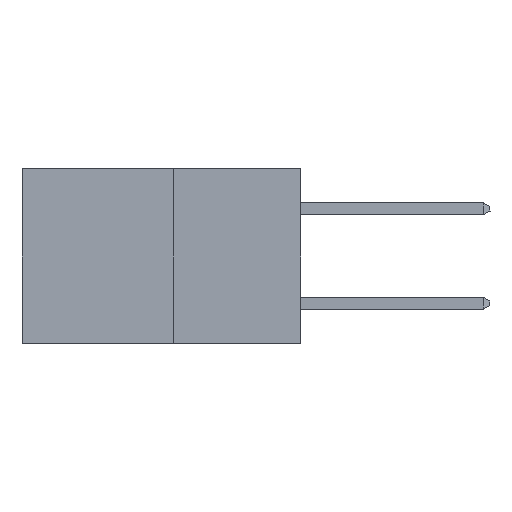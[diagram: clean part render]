
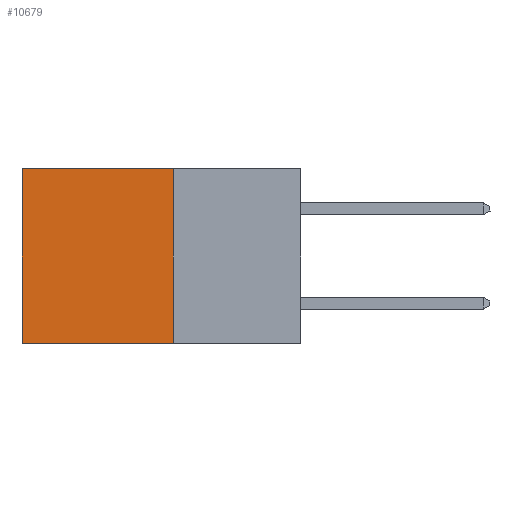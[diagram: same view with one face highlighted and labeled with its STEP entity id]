
A CAD part, left-side view. The second image highlights one B-rep face of the part: STEP entity #10679.
In plain terms, the highlighted planar face has unit normal (-1, 0, 0).
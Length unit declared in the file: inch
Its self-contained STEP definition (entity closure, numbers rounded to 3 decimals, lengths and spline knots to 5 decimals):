
#795 = DIRECTION ( 'NONE',  ( 0., 0., -1. ) ) ;
#1395 = LINE ( 'NONE', #13240, #25590 ) ;
#1588 = ORIENTED_EDGE ( 'NONE', *, *, #17756, .T. ) ;
#4269 = FACE_OUTER_BOUND ( 'NONE', #24309, .T. ) ;
#5501 = AXIS2_PLACEMENT_3D ( 'NONE', #5782, #15832, #795 ) ;
#5782 = CARTESIAN_POINT ( 'NONE',  ( 0.277, 0.27, -0.37 ) ) ;
#6312 = DIRECTION ( 'NONE',  ( 0., 0., -1. ) ) ;
#6482 = LINE ( 'NONE', #16261, #12352 ) ;
#6827 = EDGE_CURVE ( 'NONE', #15611, #18702, #25034, .T. ) ;
#7645 = DIRECTION ( 'NONE',  ( 0., 0., -1. ) ) ;
#8104 = CARTESIAN_POINT ( 'NONE',  ( 0.277, 0.27, -0.37 ) ) ;
#10357 = CARTESIAN_POINT ( 'NONE',  ( 0.277, 0.27, -0.37 ) ) ;
#10679 = ADVANCED_FACE ( 'NONE', ( #4269 ), #30623, .F. ) ;
#11931 = EDGE_CURVE ( 'NONE', #15611, #28631, #1395, .T. ) ;
#12152 = ORIENTED_EDGE ( 'NONE', *, *, #25305, .F. ) ;
#12352 = VECTOR ( 'NONE', #6312, 39.37008 ) ;
#13240 = CARTESIAN_POINT ( 'NONE',  ( 0.277, 0.27, 0. ) ) ;
#13281 = CARTESIAN_POINT ( 'NONE',  ( 0.277, 0.59, 0. ) ) ;
#15611 = VERTEX_POINT ( 'NONE', #28821 ) ;
#15832 = DIRECTION ( 'NONE',  ( 1., 0., 0. ) ) ;
#16261 = CARTESIAN_POINT ( 'NONE',  ( 0.277, 0.59, -0.37 ) ) ;
#17170 = VECTOR ( 'NONE', #20236, 39.37008 ) ;
#17756 = EDGE_CURVE ( 'NONE', #28631, #27104, #6482, .T. ) ;
#17958 = LINE ( 'NONE', #10357, #17170 ) ;
#18069 = ORIENTED_EDGE ( 'NONE', *, *, #11931, .T. ) ;
#18287 = DIRECTION ( 'NONE',  ( 0., 1., 0. ) ) ;
#18540 = ORIENTED_EDGE ( 'NONE', *, *, #6827, .F. ) ;
#18702 = VERTEX_POINT ( 'NONE', #24432 ) ;
#20011 = VECTOR ( 'NONE', #7645, 39.37008 ) ;
#20236 = DIRECTION ( 'NONE',  ( 0., 1., 0. ) ) ;
#24309 = EDGE_LOOP ( 'NONE', ( #1588, #12152, #18540, #18069 ) ) ;
#24432 = CARTESIAN_POINT ( 'NONE',  ( 0.277, 0.27, -0.37 ) ) ;
#25034 = LINE ( 'NONE', #8104, #20011 ) ;
#25305 = EDGE_CURVE ( 'NONE', #18702, #27104, #17958, .T. ) ;
#25590 = VECTOR ( 'NONE', #18287, 39.37008 ) ;
#27104 = VERTEX_POINT ( 'NONE', #32061 ) ;
#28631 = VERTEX_POINT ( 'NONE', #13281 ) ;
#28821 = CARTESIAN_POINT ( 'NONE',  ( 0.277, 0.27, 0. ) ) ;
#30623 = PLANE ( 'NONE',  #5501 ) ;
#32061 = CARTESIAN_POINT ( 'NONE',  ( 0.277, 0.59, -0.37 ) ) ;
